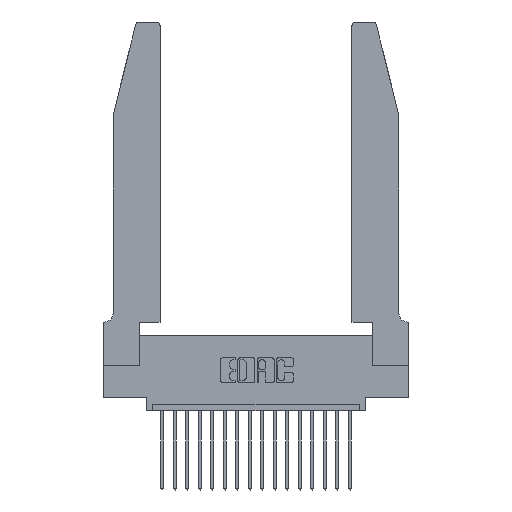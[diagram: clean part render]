
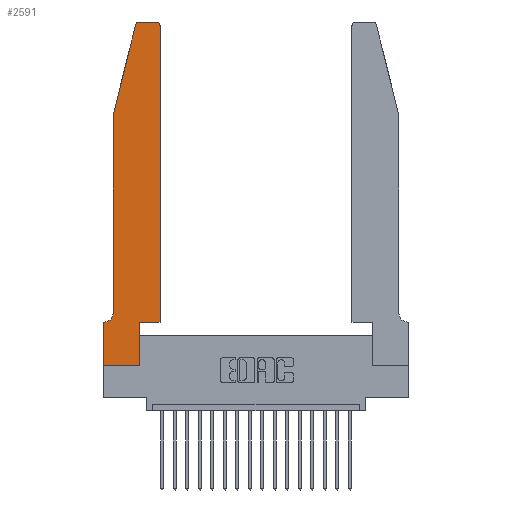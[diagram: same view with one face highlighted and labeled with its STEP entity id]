
A CAD part, top view. The second image highlights one B-rep face of the part: STEP entity #2591.
In plain terms, the highlighted planar face has unit normal (0, 0, 1).
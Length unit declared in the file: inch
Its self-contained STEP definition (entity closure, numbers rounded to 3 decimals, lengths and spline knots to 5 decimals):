
#229 = DIRECTION ( 'NONE',  ( 0., 0., 1. ) ) ;
#236 = LINE ( 'NONE', #1764, #11879 ) ;
#371 = ORIENTED_EDGE ( 'NONE', *, *, #16446, .T. ) ;
#456 = VERTEX_POINT ( 'NONE', #828 ) ;
#481 = ORIENTED_EDGE ( 'NONE', *, *, #14255, .T. ) ;
#485 = CARTESIAN_POINT ( 'NONE',  ( 0.4205, 2.75, 0.37 ) ) ;
#828 = CARTESIAN_POINT ( 'NONE',  ( 0.4505, 0.35, 0.37 ) ) ;
#1086 = DIRECTION ( 'NONE',  ( 0., 0., -1. ) ) ;
#1339 = DIRECTION ( 'NONE',  ( -0.239, -0.971, 0. ) ) ;
#1490 = LINE ( 'NONE', #6914, #12576 ) ;
#1674 = CARTESIAN_POINT ( 'NONE',  ( 0.2865, 0., 0.37 ) ) ;
#1764 = CARTESIAN_POINT ( 'NONE',  ( 0.2605, 2.75, 0.37 ) ) ;
#1974 = VERTEX_POINT ( 'NONE', #14992 ) ;
#2038 = DIRECTION ( 'NONE',  ( 0., -1., 0. ) ) ;
#2165 = ORIENTED_EDGE ( 'NONE', *, *, #3733, .T. ) ;
#2252 = CARTESIAN_POINT ( 'NONE',  ( 0.4205, 2.72, 0.37 ) ) ;
#2273 = VECTOR ( 'NONE', #17723, 39.37008 ) ;
#2411 = LINE ( 'NONE', #9894, #12276 ) ;
#2485 = EDGE_CURVE ( 'NONE', #6116, #7814, #15992, .T. ) ;
#2591 = ADVANCED_FACE ( 'NONE', ( #18494 ), #11635, .T. ) ;
#2744 = DIRECTION ( 'NONE',  ( 0., -1., 0. ) ) ;
#2983 = CARTESIAN_POINT ( 'NONE',  ( 0.2865, 0.35, 0.37 ) ) ;
#3158 = EDGE_CURVE ( 'NONE', #7527, #12712, #6457, .T. ) ;
#3196 = ORIENTED_EDGE ( 'NONE', *, *, #10362, .T. ) ;
#3493 = VERTEX_POINT ( 'NONE', #4279 ) ;
#3733 = EDGE_CURVE ( 'NONE', #1974, #16566, #9382, .T. ) ;
#3819 = LINE ( 'NONE', #9470, #6738 ) ;
#4279 = CARTESIAN_POINT ( 'NONE',  ( 0.0055, 0.35, 0.37 ) ) ;
#4586 = CARTESIAN_POINT ( 'NONE',  ( 0.0755, 0.35, 0.37 ) ) ;
#5197 = LINE ( 'NONE', #6224, #11609 ) ;
#5427 = ORIENTED_EDGE ( 'NONE', *, *, #10884, .T. ) ;
#6004 = CARTESIAN_POINT ( 'NONE',  ( 0.0055, 0.42, 0.37 ) ) ;
#6116 = VERTEX_POINT ( 'NONE', #20276 ) ;
#6224 = CARTESIAN_POINT ( 'NONE',  ( 0.4505, 0.35, 0.37 ) ) ;
#6457 = LINE ( 'NONE', #16352, #2273 ) ;
#6465 = CARTESIAN_POINT ( 'NONE',  ( 0.284, 2.72, 0.37 ) ) ;
#6616 = VERTEX_POINT ( 'NONE', #13290 ) ;
#6738 = VECTOR ( 'NONE', #1339, 39.37008 ) ;
#6838 = ORIENTED_EDGE ( 'NONE', *, *, #6885, .T. ) ;
#6885 = EDGE_CURVE ( 'NONE', #12712, #6616, #18913, .T. ) ;
#6914 = CARTESIAN_POINT ( 'NONE',  ( 0.4505, 0.35, 0.37 ) ) ;
#6917 = DIRECTION ( 'NONE',  ( 1., 0., 0. ) ) ;
#7022 = CARTESIAN_POINT ( 'NONE',  ( 0., 0.35, 0.37 ) ) ;
#7030 = CARTESIAN_POINT ( 'NONE',  ( 0.25487, 2.72718, 0.37 ) ) ;
#7527 = VERTEX_POINT ( 'NONE', #15224 ) ;
#7814 = VERTEX_POINT ( 'NONE', #7030 ) ;
#9109 = AXIS2_PLACEMENT_3D ( 'NONE', #6004, #1086, #10772 ) ;
#9118 = DIRECTION ( 'NONE',  ( -1., 0., 0. ) ) ;
#9358 = LINE ( 'NONE', #4586, #15796 ) ;
#9382 = CIRCLE ( 'NONE', #12106, 0.03 ) ;
#9470 = CARTESIAN_POINT ( 'NONE',  ( 0.0755, 2., 0.37 ) ) ;
#9574 = CARTESIAN_POINT ( 'NONE',  ( 0.0755, 2., 0.37 ) ) ;
#9894 = CARTESIAN_POINT ( 'NONE',  ( 0., 0., 0.37 ) ) ;
#10140 = VERTEX_POINT ( 'NONE', #19039 ) ;
#10226 = ORIENTED_EDGE ( 'NONE', *, *, #11672, .T. ) ;
#10257 = EDGE_LOOP ( 'NONE', ( #3196, #19510, #481, #18893, #10226, #5427, #12003, #20404, #6838, #12599, #371, #2165 ) ) ;
#10362 = EDGE_CURVE ( 'NONE', #16566, #6116, #236, .T. ) ;
#10772 = DIRECTION ( 'NONE',  ( -1., 0., 0. ) ) ;
#10884 = EDGE_CURVE ( 'NONE', #3493, #17125, #9358, .T. ) ;
#10906 = DIRECTION ( 'NONE',  ( 0., 1., 0. ) ) ;
#10970 = EDGE_CURVE ( 'NONE', #6616, #456, #5197, .T. ) ;
#11609 = VECTOR ( 'NONE', #20358, 39.37008 ) ;
#11635 = PLANE ( 'NONE',  #17885 ) ;
#11672 = EDGE_CURVE ( 'NONE', #10140, #3493, #18224, .T. ) ;
#11879 = VECTOR ( 'NONE', #12716, 39.37008 ) ;
#12003 = ORIENTED_EDGE ( 'NONE', *, *, #18231, .T. ) ;
#12106 = AXIS2_PLACEMENT_3D ( 'NONE', #2252, #16679, #13289 ) ;
#12276 = VECTOR ( 'NONE', #2038, 39.37008 ) ;
#12576 = VECTOR ( 'NONE', #17953, 39.37008 ) ;
#12599 = ORIENTED_EDGE ( 'NONE', *, *, #10970, .T. ) ;
#12712 = VERTEX_POINT ( 'NONE', #1674 ) ;
#12716 = DIRECTION ( 'NONE',  ( -1., 0., 0. ) ) ;
#12865 = VECTOR ( 'NONE', #2744, 39.37008 ) ;
#13240 = VECTOR ( 'NONE', #10906, 39.37008 ) ;
#13289 = DIRECTION ( 'NONE',  ( 1., 0., 0. ) ) ;
#13290 = CARTESIAN_POINT ( 'NONE',  ( 0.2865, 0.35, 0.37 ) ) ;
#14255 = EDGE_CURVE ( 'NONE', #7814, #19285, #3819, .T. ) ;
#14817 = CARTESIAN_POINT ( 'NONE',  ( 0., 0.35, 0.37 ) ) ;
#14992 = CARTESIAN_POINT ( 'NONE',  ( 0.4505, 2.72, 0.37 ) ) ;
#15190 = EDGE_CURVE ( 'NONE', #19285, #10140, #19314, .T. ) ;
#15224 = CARTESIAN_POINT ( 'NONE',  ( 0., 0., 0.37 ) ) ;
#15567 = CARTESIAN_POINT ( 'NONE',  ( 0.0755, 2., 0.37 ) ) ;
#15796 = VECTOR ( 'NONE', #9118, 39.37008 ) ;
#15992 = CIRCLE ( 'NONE', #18124, 0.03 ) ;
#16352 = CARTESIAN_POINT ( 'NONE',  ( 0., 0., 0.37 ) ) ;
#16383 = DIRECTION ( 'NONE',  ( 0., 0., 1. ) ) ;
#16446 = EDGE_CURVE ( 'NONE', #456, #1974, #1490, .T. ) ;
#16566 = VERTEX_POINT ( 'NONE', #485 ) ;
#16679 = DIRECTION ( 'NONE',  ( 0., 0., 1. ) ) ;
#17125 = VERTEX_POINT ( 'NONE', #7022 ) ;
#17723 = DIRECTION ( 'NONE',  ( 1., 0., 0. ) ) ;
#17885 = AXIS2_PLACEMENT_3D ( 'NONE', #14817, #16383, #6917 ) ;
#17915 = DIRECTION ( 'NONE',  ( 1., 0., 0. ) ) ;
#17953 = DIRECTION ( 'NONE',  ( 0., 1., 0. ) ) ;
#18124 = AXIS2_PLACEMENT_3D ( 'NONE', #6465, #229, #17915 ) ;
#18224 = CIRCLE ( 'NONE', #9109, 0.07 ) ;
#18231 = EDGE_CURVE ( 'NONE', #17125, #7527, #2411, .T. ) ;
#18494 = FACE_OUTER_BOUND ( 'NONE', #10257, .T. ) ;
#18893 = ORIENTED_EDGE ( 'NONE', *, *, #15190, .T. ) ;
#18913 = LINE ( 'NONE', #2983, #13240 ) ;
#19039 = CARTESIAN_POINT ( 'NONE',  ( 0.0755, 0.42, 0.37 ) ) ;
#19285 = VERTEX_POINT ( 'NONE', #9574 ) ;
#19314 = LINE ( 'NONE', #15567, #12865 ) ;
#19510 = ORIENTED_EDGE ( 'NONE', *, *, #2485, .T. ) ;
#20276 = CARTESIAN_POINT ( 'NONE',  ( 0.284, 2.75, 0.37 ) ) ;
#20358 = DIRECTION ( 'NONE',  ( 1., 0., 0. ) ) ;
#20404 = ORIENTED_EDGE ( 'NONE', *, *, #3158, .T. ) ;
